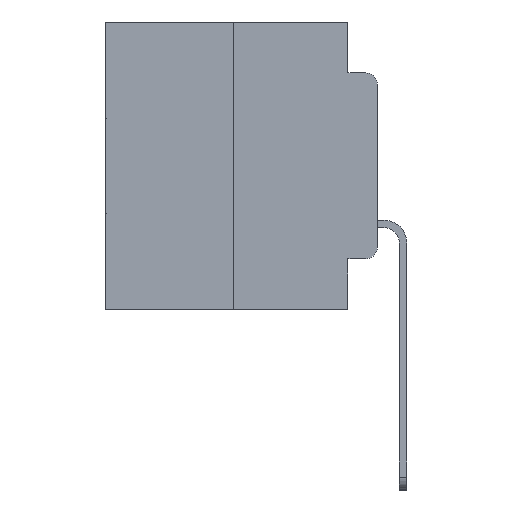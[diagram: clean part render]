
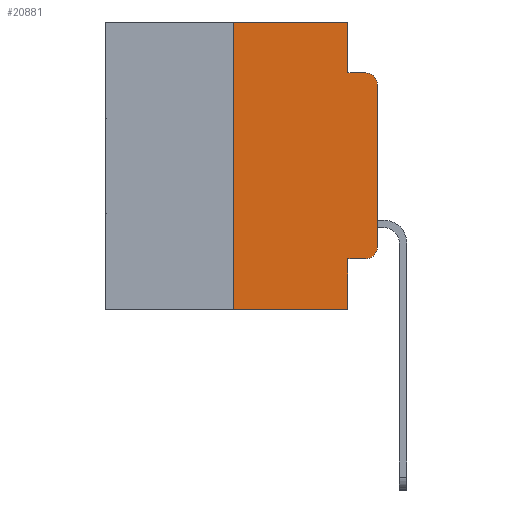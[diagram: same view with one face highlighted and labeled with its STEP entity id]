
A CAD part, left-side view. The second image highlights one B-rep face of the part: STEP entity #20881.
In plain terms, the highlighted planar face has unit normal (-1, 0, 0).
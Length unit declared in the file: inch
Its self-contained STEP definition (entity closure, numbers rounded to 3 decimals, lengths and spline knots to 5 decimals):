
#248 = CARTESIAN_POINT ( 'NONE',  ( 0., 0., -0.1085 ) ) ;
#284 = ORIENTED_EDGE ( 'NONE', *, *, #22583, .T. ) ;
#1253 = CARTESIAN_POINT ( 'NONE',  ( 0., 0.051, 0. ) ) ;
#1445 = LINE ( 'NONE', #2282, #2187 ) ;
#2187 = VECTOR ( 'NONE', #18152, 39.37008 ) ;
#2282 = CARTESIAN_POINT ( 'NONE',  ( 0., 0.473, -0.5 ) ) ;
#2397 = EDGE_CURVE ( 'NONE', #13105, #28851, #26145, .T. ) ;
#2517 = ORIENTED_EDGE ( 'NONE', *, *, #13786, .T. ) ;
#2957 = ORIENTED_EDGE ( 'NONE', *, *, #28774, .F. ) ;
#3687 = VERTEX_POINT ( 'NONE', #28357 ) ;
#4065 = LINE ( 'NONE', #24410, #15434 ) ;
#4530 = VERTEX_POINT ( 'NONE', #22929 ) ;
#5047 = CARTESIAN_POINT ( 'NONE',  ( 0., 0.25, 0. ) ) ;
#5913 = CARTESIAN_POINT ( 'NONE',  ( 0., 0.473, 0. ) ) ;
#6211 = AXIS2_PLACEMENT_3D ( 'NONE', #28304, #26127, #19630 ) ;
#6508 = VERTEX_POINT ( 'NONE', #5047 ) ;
#7439 = VERTEX_POINT ( 'NONE', #27902 ) ;
#7697 = EDGE_CURVE ( 'NONE', #12287, #4530, #9198, .T. ) ;
#8244 = DIRECTION ( 'NONE',  ( 0., -1., 0. ) ) ;
#8812 = CARTESIAN_POINT ( 'NONE',  ( 0., 0., -0.3915 ) ) ;
#9198 = LINE ( 'NONE', #22295, #25455 ) ;
#10298 = FACE_OUTER_BOUND ( 'NONE', #15970, .T. ) ;
#11046 = CARTESIAN_POINT ( 'NONE',  ( 0., 0.02, -0.1085 ) ) ;
#11606 = ORIENTED_EDGE ( 'NONE', *, *, #17656, .F. ) ;
#12090 = CARTESIAN_POINT ( 'NONE',  ( 0., 0.02, -0.3915 ) ) ;
#12148 = AXIS2_PLACEMENT_3D ( 'NONE', #12090, #27484, #14352 ) ;
#12287 = VERTEX_POINT ( 'NONE', #23904 ) ;
#13105 = VERTEX_POINT ( 'NONE', #248 ) ;
#13260 = DIRECTION ( 'NONE',  ( 0., 0., -1. ) ) ;
#13427 = DIRECTION ( 'NONE',  ( 0., 0., 1. ) ) ;
#13514 = VERTEX_POINT ( 'NONE', #17675 ) ;
#13786 = EDGE_CURVE ( 'NONE', #7439, #24535, #20776, .T. ) ;
#14352 = DIRECTION ( 'NONE',  ( 0., 0., -1. ) ) ;
#14574 = EDGE_CURVE ( 'NONE', #6508, #12287, #22781, .T. ) ;
#15205 = CARTESIAN_POINT ( 'NONE',  ( 0., 0.02, -0.0885 ) ) ;
#15434 = VECTOR ( 'NONE', #13427, 39.37008 ) ;
#15662 = DIRECTION ( 'NONE',  ( 0., 0., -1. ) ) ;
#15791 = ORIENTED_EDGE ( 'NONE', *, *, #27802, .T. ) ;
#15970 = EDGE_LOOP ( 'NONE', ( #284, #23173, #2957, #26299, #24057, #11606, #15791, #15987, #28433, #2517 ) ) ;
#15987 = ORIENTED_EDGE ( 'NONE', *, *, #24995, .F. ) ;
#16038 = VECTOR ( 'NONE', #8244, 39.37008 ) ;
#16097 = VECTOR ( 'NONE', #19407, 39.37008 ) ;
#16180 = AXIS2_PLACEMENT_3D ( 'NONE', #11046, #26439, #13260 ) ;
#16261 = VECTOR ( 'NONE', #21561, 39.37008 ) ;
#16732 = LINE ( 'NONE', #28040, #16038 ) ;
#16945 = CARTESIAN_POINT ( 'NONE',  ( 0., 0.051, -0.4115 ) ) ;
#17426 = PLANE ( 'NONE',  #6211 ) ;
#17656 = EDGE_CURVE ( 'NONE', #3687, #6508, #24677, .T. ) ;
#17675 = CARTESIAN_POINT ( 'NONE',  ( 0., 0.051, -0.5 ) ) ;
#18152 = DIRECTION ( 'NONE',  ( 0., -1., 0. ) ) ;
#18722 = CARTESIAN_POINT ( 'NONE',  ( 0., 0.25, 0. ) ) ;
#18995 = VERTEX_POINT ( 'NONE', #16945 ) ;
#19401 = DIRECTION ( 'NONE',  ( 0., 0., -1. ) ) ;
#19407 = DIRECTION ( 'NONE',  ( 0., -1., 0. ) ) ;
#19630 = DIRECTION ( 'NONE',  ( 0., 0., -1. ) ) ;
#20057 = VECTOR ( 'NONE', #19401, 39.37008 ) ;
#20738 = LINE ( 'NONE', #1253, #20057 ) ;
#20776 = CIRCLE ( 'NONE', #12148, 0.02 ) ;
#20881 = ADVANCED_FACE ( 'NONE', ( #10298 ), #17426, .F. ) ;
#21561 = DIRECTION ( 'NONE',  ( 0., -1., 0. ) ) ;
#22295 = CARTESIAN_POINT ( 'NONE',  ( 0., 0.051, 0. ) ) ;
#22583 = EDGE_CURVE ( 'NONE', #24535, #13105, #4065, .T. ) ;
#22626 = LINE ( 'NONE', #23724, #16097 ) ;
#22781 = LINE ( 'NONE', #5913, #16261 ) ;
#22929 = CARTESIAN_POINT ( 'NONE',  ( 0., 0.051, -0.0885 ) ) ;
#22977 = EDGE_CURVE ( 'NONE', #18995, #7439, #22626, .T. ) ;
#23137 = DIRECTION ( 'NONE',  ( 0., 0., 1. ) ) ;
#23173 = ORIENTED_EDGE ( 'NONE', *, *, #2397, .T. ) ;
#23724 = CARTESIAN_POINT ( 'NONE',  ( 0., 0.051, -0.4115 ) ) ;
#23904 = CARTESIAN_POINT ( 'NONE',  ( 0., 0.051, 0. ) ) ;
#24007 = VECTOR ( 'NONE', #23137, 39.37008 ) ;
#24057 = ORIENTED_EDGE ( 'NONE', *, *, #14574, .F. ) ;
#24410 = CARTESIAN_POINT ( 'NONE',  ( 0., 0., 0. ) ) ;
#24535 = VERTEX_POINT ( 'NONE', #8812 ) ;
#24677 = LINE ( 'NONE', #18722, #24007 ) ;
#24995 = EDGE_CURVE ( 'NONE', #18995, #13514, #20738, .T. ) ;
#25455 = VECTOR ( 'NONE', #15662, 39.37008 ) ;
#26127 = DIRECTION ( 'NONE',  ( 1., 0., 0. ) ) ;
#26145 = CIRCLE ( 'NONE', #16180, 0.02 ) ;
#26299 = ORIENTED_EDGE ( 'NONE', *, *, #7697, .F. ) ;
#26439 = DIRECTION ( 'NONE',  ( -1., 0., 0. ) ) ;
#27484 = DIRECTION ( 'NONE',  ( -1., 0., 0. ) ) ;
#27802 = EDGE_CURVE ( 'NONE', #3687, #13514, #1445, .T. ) ;
#27902 = CARTESIAN_POINT ( 'NONE',  ( 0., 0.02, -0.4115 ) ) ;
#28040 = CARTESIAN_POINT ( 'NONE',  ( 0., 0.051, -0.0885 ) ) ;
#28304 = CARTESIAN_POINT ( 'NONE',  ( 0., 0.473, 0. ) ) ;
#28357 = CARTESIAN_POINT ( 'NONE',  ( 0., 0.25, -0.5 ) ) ;
#28433 = ORIENTED_EDGE ( 'NONE', *, *, #22977, .T. ) ;
#28774 = EDGE_CURVE ( 'NONE', #4530, #28851, #16732, .T. ) ;
#28851 = VERTEX_POINT ( 'NONE', #15205 ) ;
